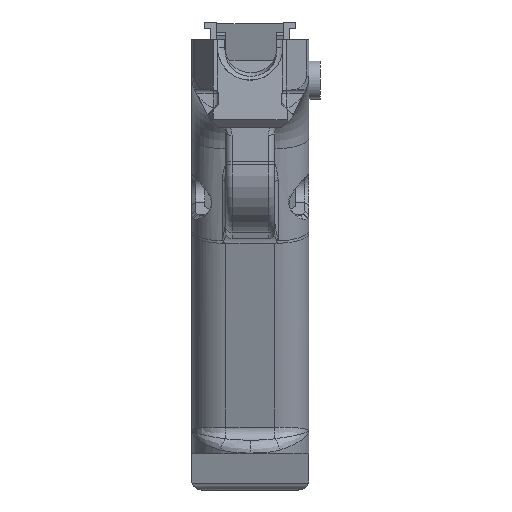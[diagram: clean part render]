
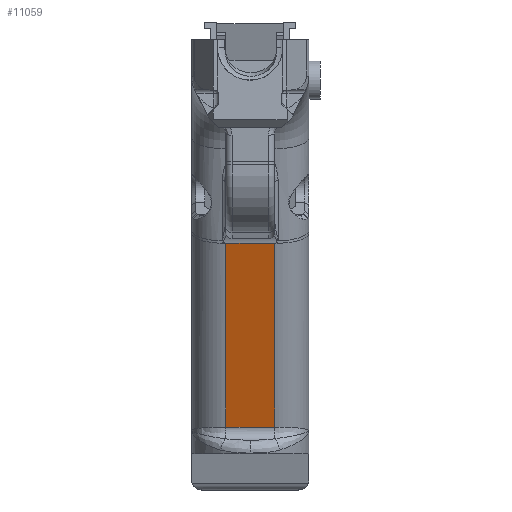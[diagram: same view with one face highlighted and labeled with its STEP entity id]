
A CAD part, front view. The second image highlights one B-rep face of the part: STEP entity #11059.
In plain terms, the highlighted planar face has unit normal (0, -0.947, -0.322).
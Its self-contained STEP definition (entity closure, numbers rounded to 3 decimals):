
#1192=FACE_OUTER_BOUND('',#1809,.T.);
#1809=EDGE_LOOP('',(#9325,#9326,#9327,#9328));
#2326=LINE('',#15601,#3489);
#3012=LINE('',#18801,#4175);
#3013=LINE('',#18821,#4176);
#3014=LINE('',#18822,#4177);
#3489=VECTOR('',#12795,10.);
#4175=VECTOR('',#14285,10.);
#4176=VECTOR('',#14290,10.);
#4177=VECTOR('',#14291,10.);
#4557=VERTEX_POINT('',#15598);
#4558=VERTEX_POINT('',#15600);
#5204=VERTEX_POINT('',#18793);
#5205=VERTEX_POINT('',#18800);
#5737=EDGE_CURVE('',#4557,#4558,#2326,.T.);
#6668=EDGE_CURVE('',#5204,#5205,#3012,.T.);
#6672=EDGE_CURVE('',#5205,#4557,#3013,.T.);
#6673=EDGE_CURVE('',#4558,#5204,#3014,.T.);
#9325=ORIENTED_EDGE('',*,*,#6672,.F.);
#9326=ORIENTED_EDGE('',*,*,#6668,.F.);
#9327=ORIENTED_EDGE('',*,*,#6673,.F.);
#9328=ORIENTED_EDGE('',*,*,#5737,.F.);
#10585=PLANE('',#11906);
#11059=ADVANCED_FACE('',(#1192),#10585,.T.);
#11906=AXIS2_PLACEMENT_3D('',#18820,#14288,#14289);
#12795=DIRECTION('',(0.,-0.322,0.947));
#14285=DIRECTION('',(0.,0.322,-0.947));
#14288=DIRECTION('center_axis',(0.,-0.947,-0.322));
#14289=DIRECTION('ref_axis',(0.,0.322,-0.947));
#14290=DIRECTION('',(-1.,0.,0.));
#14291=DIRECTION('',(1.,0.,0.));
#15598=CARTESIAN_POINT('',(-14.218,-62.644,-85.79));
#15600=CARTESIAN_POINT('',(-14.218,-78.109,-40.345));
#15601=CARTESIAN_POINT('',(-14.218,-83.303,-25.083));
#18793=CARTESIAN_POINT('',(-2.118,-78.109,-40.345));
#18800=CARTESIAN_POINT('',(-2.118,-62.644,-85.79));
#18801=CARTESIAN_POINT('',(-2.118,-83.303,-25.083));
#18820=CARTESIAN_POINT('Origin',(-22.668,-78.109,-40.345));
#18821=CARTESIAN_POINT('',(-15.418,-62.644,-85.79));
#18822=CARTESIAN_POINT('',(0.,-78.109,-40.345));
